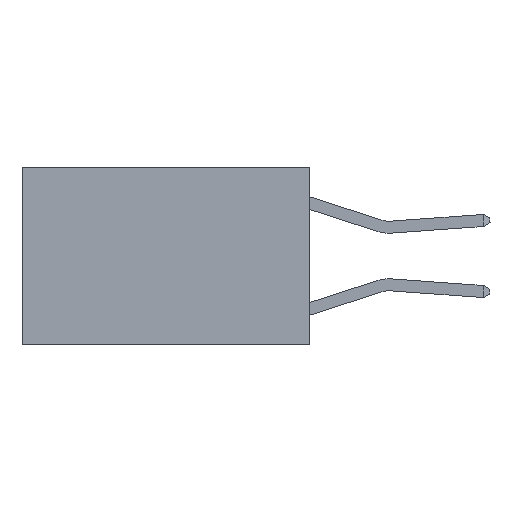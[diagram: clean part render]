
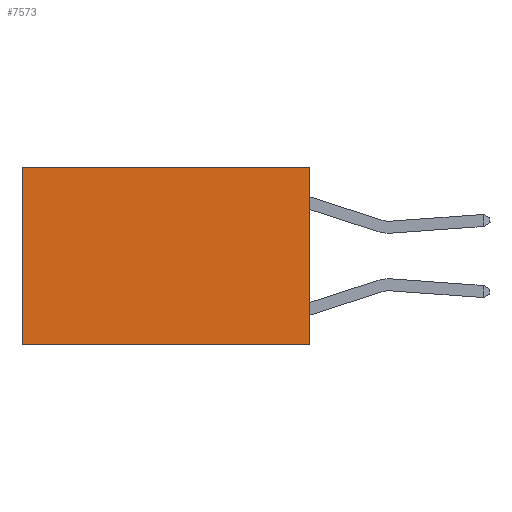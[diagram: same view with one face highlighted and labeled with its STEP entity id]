
A CAD part, left-side view. The second image highlights one B-rep face of the part: STEP entity #7573.
In plain terms, the highlighted planar face has unit normal (-1, 0, 0).
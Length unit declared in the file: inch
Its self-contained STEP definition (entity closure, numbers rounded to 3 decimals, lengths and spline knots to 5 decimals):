
#1630 = LINE ( 'NONE', #7768, #4557 ) ;
#1820 = DIRECTION ( 'NONE',  ( 0., 0., -1. ) ) ;
#2499 = ORIENTED_EDGE ( 'NONE', *, *, #10932, .T. ) ;
#2520 = VERTEX_POINT ( 'NONE', #3423 ) ;
#3014 = DIRECTION ( 'NONE',  ( 0., 1., 0. ) ) ;
#3118 = VERTEX_POINT ( 'NONE', #11115 ) ;
#3174 = CARTESIAN_POINT ( 'NONE',  ( 0.2625, 0.6, 0. ) ) ;
#3423 = CARTESIAN_POINT ( 'NONE',  ( 0.2625, 0.6, -0.37 ) ) ;
#4190 = CARTESIAN_POINT ( 'NONE',  ( 0.2625, 0., -0.37 ) ) ;
#4362 = VECTOR ( 'NONE', #6207, 39.37008 ) ;
#4504 = CARTESIAN_POINT ( 'NONE',  ( 0.2625, 0., 0. ) ) ;
#4557 = VECTOR ( 'NONE', #1820, 39.37008 ) ;
#5409 = FACE_OUTER_BOUND ( 'NONE', #7661, .T. ) ;
#5507 = DIRECTION ( 'NONE',  ( 0., 0., -1. ) ) ;
#5882 = CARTESIAN_POINT ( 'NONE',  ( 0.2625, 0., 0. ) ) ;
#5948 = EDGE_CURVE ( 'NONE', #11120, #2520, #8556, .T. ) ;
#6038 = EDGE_CURVE ( 'NONE', #8044, #2520, #6712, .T. ) ;
#6207 = DIRECTION ( 'NONE',  ( 0., 0., -1. ) ) ;
#6712 = LINE ( 'NONE', #12090, #4362 ) ;
#6985 = CARTESIAN_POINT ( 'NONE',  ( 0.2625, 0., -0.37 ) ) ;
#7300 = AXIS2_PLACEMENT_3D ( 'NONE', #4504, #11412, #5507 ) ;
#7573 = ADVANCED_FACE ( 'NONE', ( #5409 ), #11362, .F. ) ;
#7661 = EDGE_LOOP ( 'NONE', ( #9445, #9746, #12670, #2499 ) ) ;
#7768 = CARTESIAN_POINT ( 'NONE',  ( 0.2625, 0., 0. ) ) ;
#8044 = VERTEX_POINT ( 'NONE', #3174 ) ;
#8247 = VECTOR ( 'NONE', #3014, 39.37008 ) ;
#8432 = LINE ( 'NONE', #5882, #10720 ) ;
#8556 = LINE ( 'NONE', #6985, #8247 ) ;
#9445 = ORIENTED_EDGE ( 'NONE', *, *, #6038, .T. ) ;
#9746 = ORIENTED_EDGE ( 'NONE', *, *, #5948, .F. ) ;
#10132 = EDGE_CURVE ( 'NONE', #3118, #11120, #1630, .T. ) ;
#10720 = VECTOR ( 'NONE', #10788, 39.37008 ) ;
#10788 = DIRECTION ( 'NONE',  ( 0., 1., 0. ) ) ;
#10932 = EDGE_CURVE ( 'NONE', #3118, #8044, #8432, .T. ) ;
#11115 = CARTESIAN_POINT ( 'NONE',  ( 0.2625, 0., 0. ) ) ;
#11120 = VERTEX_POINT ( 'NONE', #4190 ) ;
#11362 = PLANE ( 'NONE',  #7300 ) ;
#11412 = DIRECTION ( 'NONE',  ( 1., 0., 0. ) ) ;
#12090 = CARTESIAN_POINT ( 'NONE',  ( 0.2625, 0.6, 0. ) ) ;
#12670 = ORIENTED_EDGE ( 'NONE', *, *, #10132, .F. ) ;
